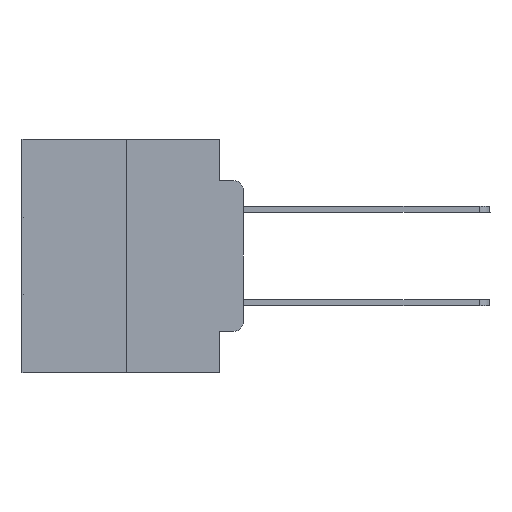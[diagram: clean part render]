
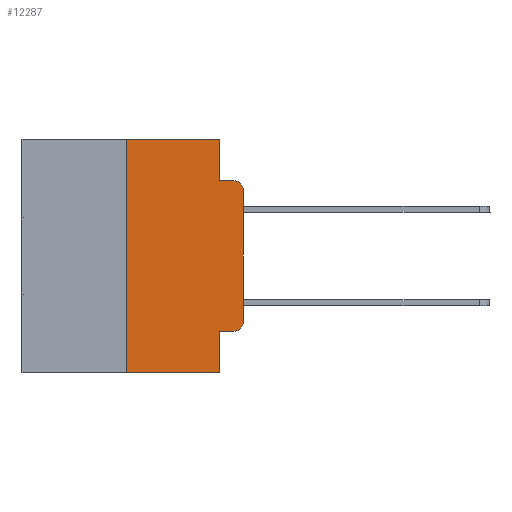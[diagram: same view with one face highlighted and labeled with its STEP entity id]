
A CAD part, left-side view. The second image highlights one B-rep face of the part: STEP entity #12287.
In plain terms, the highlighted planar face has unit normal (-1, 0, 0).
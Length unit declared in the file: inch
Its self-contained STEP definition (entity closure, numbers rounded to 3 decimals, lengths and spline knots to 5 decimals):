
#78 = DIRECTION ( 'NONE',  ( 0., 0., -1. ) ) ;
#397 = VECTOR ( 'NONE', #11625, 39.37008 ) ;
#619 = CIRCLE ( 'NONE', #1131, 0.02 ) ;
#630 = CARTESIAN_POINT ( 'NONE',  ( 0., 0.051, 0. ) ) ;
#650 = CARTESIAN_POINT ( 'NONE',  ( 0., 0.02, -0.3915 ) ) ;
#946 = LINE ( 'NONE', #17291, #23433 ) ;
#1131 = AXIS2_PLACEMENT_3D ( 'NONE', #12308, #10140, #3140 ) ;
#1178 = LINE ( 'NONE', #28560, #10389 ) ;
#1550 = ORIENTED_EDGE ( 'NONE', *, *, #27508, .T. ) ;
#2700 = LINE ( 'NONE', #23182, #13758 ) ;
#2796 = VECTOR ( 'NONE', #21398, 39.37008 ) ;
#3140 = DIRECTION ( 'NONE',  ( 0., 0., -1. ) ) ;
#3367 = ORIENTED_EDGE ( 'NONE', *, *, #9132, .T. ) ;
#3750 = CARTESIAN_POINT ( 'NONE',  ( 0., 0., -0.3915 ) ) ;
#4204 = ORIENTED_EDGE ( 'NONE', *, *, #22276, .T. ) ;
#4664 = ORIENTED_EDGE ( 'NONE', *, *, #24726, .F. ) ;
#5449 = VECTOR ( 'NONE', #28314, 39.37008 ) ;
#5510 = VERTEX_POINT ( 'NONE', #14819 ) ;
#6865 = CARTESIAN_POINT ( 'NONE',  ( 0., 0., 0. ) ) ;
#7491 = DIRECTION ( 'NONE',  ( 0., -1., 0. ) ) ;
#8529 = ORIENTED_EDGE ( 'NONE', *, *, #27361, .F. ) ;
#8763 = ORIENTED_EDGE ( 'NONE', *, *, #13821, .F. ) ;
#9132 = EDGE_CURVE ( 'NONE', #12004, #20195, #30183, .T. ) ;
#9140 = LINE ( 'NONE', #21034, #5449 ) ;
#9763 = FACE_OUTER_BOUND ( 'NONE', #29351, .T. ) ;
#10140 = DIRECTION ( 'NONE',  ( -1., 0., 0. ) ) ;
#10389 = VECTOR ( 'NONE', #21391, 39.37008 ) ;
#10491 = AXIS2_PLACEMENT_3D ( 'NONE', #650, #21707, #24049 ) ;
#10746 = CARTESIAN_POINT ( 'NONE',  ( 0., 0.051, -0.0885 ) ) ;
#11625 = DIRECTION ( 'NONE',  ( 0., 0., 1. ) ) ;
#12004 = VERTEX_POINT ( 'NONE', #3750 ) ;
#12112 = DIRECTION ( 'NONE',  ( 1., 0., 0. ) ) ;
#12287 = ADVANCED_FACE ( 'NONE', ( #9763 ), #21045, .F. ) ;
#12308 = CARTESIAN_POINT ( 'NONE',  ( 0., 0.02, -0.1085 ) ) ;
#13471 = VECTOR ( 'NONE', #17075, 39.37008 ) ;
#13500 = LINE ( 'NONE', #630, #13471 ) ;
#13523 = VERTEX_POINT ( 'NONE', #21725 ) ;
#13758 = VECTOR ( 'NONE', #30358, 39.37008 ) ;
#13821 = EDGE_CURVE ( 'NONE', #18727, #17372, #20084, .T. ) ;
#13934 = AXIS2_PLACEMENT_3D ( 'NONE', #16405, #12112, #78 ) ;
#14499 = CARTESIAN_POINT ( 'NONE',  ( 0., 0.473, 0. ) ) ;
#14614 = ORIENTED_EDGE ( 'NONE', *, *, #27445, .F. ) ;
#14819 = CARTESIAN_POINT ( 'NONE',  ( 0., 0.02, -0.0885 ) ) ;
#15650 = CARTESIAN_POINT ( 'NONE',  ( 0., 0.051, 0. ) ) ;
#16359 = VERTEX_POINT ( 'NONE', #28555 ) ;
#16405 = CARTESIAN_POINT ( 'NONE',  ( 0., 0.473, 0. ) ) ;
#17075 = DIRECTION ( 'NONE',  ( 0., 0., -1. ) ) ;
#17291 = CARTESIAN_POINT ( 'NONE',  ( 0., 0.051, -0.4115 ) ) ;
#17372 = VERTEX_POINT ( 'NONE', #10746 ) ;
#17537 = LINE ( 'NONE', #14499, #2796 ) ;
#17654 = EDGE_CURVE ( 'NONE', #25802, #12004, #29068, .T. ) ;
#18122 = CARTESIAN_POINT ( 'NONE',  ( 0., 0.051, -0.4115 ) ) ;
#18727 = VERTEX_POINT ( 'NONE', #30222 ) ;
#19294 = EDGE_CURVE ( 'NONE', #20337, #16359, #9140, .T. ) ;
#19324 = CARTESIAN_POINT ( 'NONE',  ( 0., 0., -0.1085 ) ) ;
#20084 = LINE ( 'NONE', #15650, #26353 ) ;
#20195 = VERTEX_POINT ( 'NONE', #19324 ) ;
#20337 = VERTEX_POINT ( 'NONE', #26931 ) ;
#21034 = CARTESIAN_POINT ( 'NONE',  ( 0., 0.473, -0.5 ) ) ;
#21045 = PLANE ( 'NONE',  #13934 ) ;
#21391 = DIRECTION ( 'NONE',  ( 0., 0., 1. ) ) ;
#21398 = DIRECTION ( 'NONE',  ( 0., -1., 0. ) ) ;
#21707 = DIRECTION ( 'NONE',  ( -1., 0., 0. ) ) ;
#21725 = CARTESIAN_POINT ( 'NONE',  ( 0., 0.25, 0. ) ) ;
#22276 = EDGE_CURVE ( 'NONE', #20195, #5510, #619, .T. ) ;
#23182 = CARTESIAN_POINT ( 'NONE',  ( 0., 0.051, -0.0885 ) ) ;
#23433 = VECTOR ( 'NONE', #7491, 39.37008 ) ;
#24049 = DIRECTION ( 'NONE',  ( 0., 0., -1. ) ) ;
#24726 = EDGE_CURVE ( 'NONE', #17372, #5510, #2700, .T. ) ;
#24788 = DIRECTION ( 'NONE',  ( 0., 0., -1. ) ) ;
#25613 = EDGE_CURVE ( 'NONE', #20337, #13523, #1178, .T. ) ;
#25802 = VERTEX_POINT ( 'NONE', #29588 ) ;
#26353 = VECTOR ( 'NONE', #24788, 39.37008 ) ;
#26931 = CARTESIAN_POINT ( 'NONE',  ( 0., 0.25, -0.5 ) ) ;
#27190 = ORIENTED_EDGE ( 'NONE', *, *, #19294, .T. ) ;
#27361 = EDGE_CURVE ( 'NONE', #13523, #18727, #17537, .T. ) ;
#27445 = EDGE_CURVE ( 'NONE', #30240, #16359, #13500, .T. ) ;
#27508 = EDGE_CURVE ( 'NONE', #30240, #25802, #946, .T. ) ;
#28314 = DIRECTION ( 'NONE',  ( 0., -1., 0. ) ) ;
#28555 = CARTESIAN_POINT ( 'NONE',  ( 0., 0.051, -0.5 ) ) ;
#28560 = CARTESIAN_POINT ( 'NONE',  ( 0., 0.25, 0. ) ) ;
#29068 = CIRCLE ( 'NONE', #10491, 0.02 ) ;
#29082 = ORIENTED_EDGE ( 'NONE', *, *, #25613, .F. ) ;
#29351 = EDGE_LOOP ( 'NONE', ( #3367, #4204, #4664, #8763, #8529, #29082, #27190, #14614, #1550, #30342 ) ) ;
#29588 = CARTESIAN_POINT ( 'NONE',  ( 0., 0.02, -0.4115 ) ) ;
#30183 = LINE ( 'NONE', #6865, #397 ) ;
#30222 = CARTESIAN_POINT ( 'NONE',  ( 0., 0.051, 0. ) ) ;
#30240 = VERTEX_POINT ( 'NONE', #18122 ) ;
#30342 = ORIENTED_EDGE ( 'NONE', *, *, #17654, .T. ) ;
#30358 = DIRECTION ( 'NONE',  ( 0., -1., 0. ) ) ;
